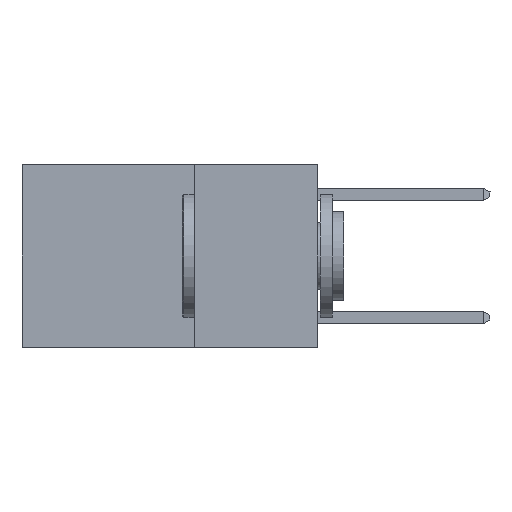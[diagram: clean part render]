
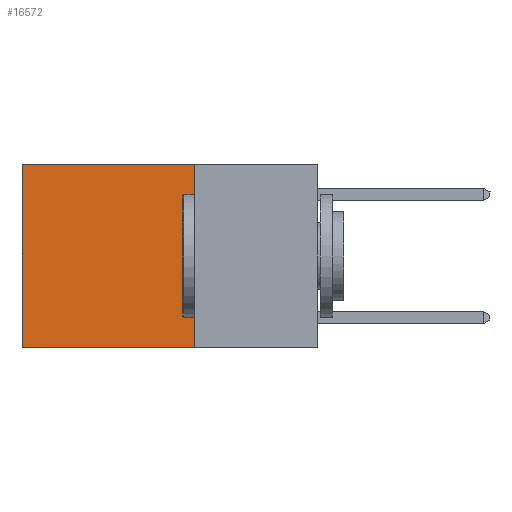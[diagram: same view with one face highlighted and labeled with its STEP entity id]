
A CAD part, left-side view. The second image highlights one B-rep face of the part: STEP entity #16572.
In plain terms, the highlighted planar face has unit normal (-1, 0, 0).
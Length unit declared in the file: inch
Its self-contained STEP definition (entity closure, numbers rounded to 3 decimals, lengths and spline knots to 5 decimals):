
#225 = DIRECTION ( 'NONE',  ( 1., 0., 0. ) ) ;
#334 = LINE ( 'NONE', #7450, #4664 ) ;
#1336 = LINE ( 'NONE', #19597, #14913 ) ;
#1971 = CARTESIAN_POINT ( 'NONE',  ( 0.2625, 0.25, -0.37 ) ) ;
#2006 = PLANE ( 'NONE',  #12865 ) ;
#4309 = DIRECTION ( 'NONE',  ( 0., 0., -1. ) ) ;
#4664 = VECTOR ( 'NONE', #18571, 39.37008 ) ;
#4720 = DIRECTION ( 'NONE',  ( 0., 1., 0. ) ) ;
#6615 = VERTEX_POINT ( 'NONE', #8024 ) ;
#6680 = VECTOR ( 'NONE', #4309, 39.37008 ) ;
#7450 = CARTESIAN_POINT ( 'NONE',  ( 0.2625, 0.25, 0. ) ) ;
#7865 = CARTESIAN_POINT ( 'NONE',  ( 0.2625, 0.6, -0.37 ) ) ;
#8024 = CARTESIAN_POINT ( 'NONE',  ( 0.2625, 0.6, 0. ) ) ;
#8784 = DIRECTION ( 'NONE',  ( 0., 0., -1. ) ) ;
#8933 = ORIENTED_EDGE ( 'NONE', *, *, #19527, .T. ) ;
#8951 = VECTOR ( 'NONE', #8784, 39.37008 ) ;
#9069 = ORIENTED_EDGE ( 'NONE', *, *, #14984, .F. ) ;
#9522 = ORIENTED_EDGE ( 'NONE', *, *, #23108, .F. ) ;
#10375 = VERTEX_POINT ( 'NONE', #1971 ) ;
#12368 = CARTESIAN_POINT ( 'NONE',  ( 0.2625, 0.25, 0. ) ) ;
#12865 = AXIS2_PLACEMENT_3D ( 'NONE', #13082, #225, #13161 ) ;
#13082 = CARTESIAN_POINT ( 'NONE',  ( 0.2625, 0.25, 0. ) ) ;
#13161 = DIRECTION ( 'NONE',  ( 0., 0., -1. ) ) ;
#13655 = VERTEX_POINT ( 'NONE', #7865 ) ;
#14013 = EDGE_LOOP ( 'NONE', ( #8933, #9522, #9069, #17074 ) ) ;
#14256 = VERTEX_POINT ( 'NONE', #12368 ) ;
#14913 = VECTOR ( 'NONE', #4720, 39.37008 ) ;
#14984 = EDGE_CURVE ( 'NONE', #14256, #10375, #19924, .T. ) ;
#15355 = CARTESIAN_POINT ( 'NONE',  ( 0.2625, 0.6, 0. ) ) ;
#16572 = ADVANCED_FACE ( 'NONE', ( #20706 ), #2006, .F. ) ;
#17074 = ORIENTED_EDGE ( 'NONE', *, *, #20084, .T. ) ;
#17964 = CARTESIAN_POINT ( 'NONE',  ( 0.2625, 0.25, 0. ) ) ;
#18571 = DIRECTION ( 'NONE',  ( 0., 1., 0. ) ) ;
#19527 = EDGE_CURVE ( 'NONE', #6615, #13655, #20851, .T. ) ;
#19597 = CARTESIAN_POINT ( 'NONE',  ( 0.2625, 0.25, -0.37 ) ) ;
#19924 = LINE ( 'NONE', #17964, #8951 ) ;
#20084 = EDGE_CURVE ( 'NONE', #14256, #6615, #334, .T. ) ;
#20706 = FACE_OUTER_BOUND ( 'NONE', #14013, .T. ) ;
#20851 = LINE ( 'NONE', #15355, #6680 ) ;
#23108 = EDGE_CURVE ( 'NONE', #10375, #13655, #1336, .T. ) ;
